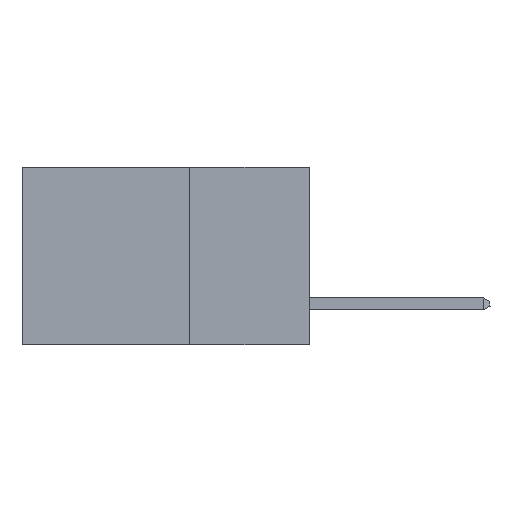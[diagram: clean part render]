
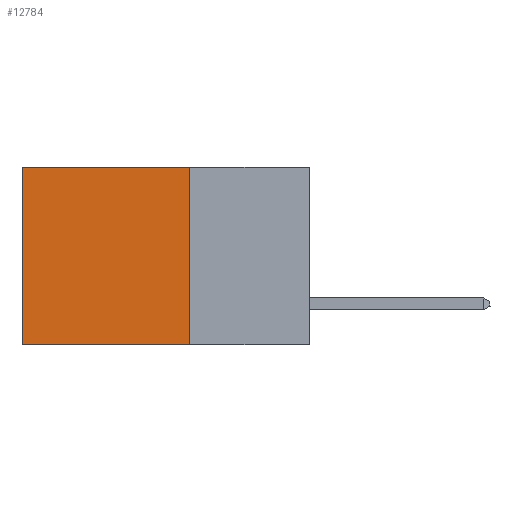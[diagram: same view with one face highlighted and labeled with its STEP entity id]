
A CAD part, left-side view. The second image highlights one B-rep face of the part: STEP entity #12784.
In plain terms, the highlighted planar face has unit normal (-1, 0, 0).
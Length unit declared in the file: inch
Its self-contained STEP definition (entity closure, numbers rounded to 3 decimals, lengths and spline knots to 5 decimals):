
#318 = EDGE_CURVE ( 'NONE', #12839, #1409, #3065, .T. ) ;
#541 = VECTOR ( 'NONE', #3881, 39.37008 ) ;
#1409 = VERTEX_POINT ( 'NONE', #2378 ) ;
#1896 = DIRECTION ( 'NONE',  ( 0., 1., 0. ) ) ;
#2196 = CARTESIAN_POINT ( 'NONE',  ( 0.2875, 0.25, 0. ) ) ;
#2378 = CARTESIAN_POINT ( 'NONE',  ( 0.2875, 0.6, -0.37 ) ) ;
#2907 = LINE ( 'NONE', #13317, #11770 ) ;
#3065 = LINE ( 'NONE', #16503, #20338 ) ;
#3502 = EDGE_LOOP ( 'NONE', ( #15024, #5044, #19921, #14026 ) ) ;
#3881 = DIRECTION ( 'NONE',  ( 0., 0., -1. ) ) ;
#5044 = ORIENTED_EDGE ( 'NONE', *, *, #7681, .F. ) ;
#6520 = DIRECTION ( 'NONE',  ( 0., 0., -1. ) ) ;
#7225 = AXIS2_PLACEMENT_3D ( 'NONE', #13760, #9853, #7696 ) ;
#7401 = LINE ( 'NONE', #12942, #8440 ) ;
#7681 = EDGE_CURVE ( 'NONE', #14162, #1409, #7401, .T. ) ;
#7696 = DIRECTION ( 'NONE',  ( 0., 0., -1. ) ) ;
#8440 = VECTOR ( 'NONE', #1896, 39.37008 ) ;
#9853 = DIRECTION ( 'NONE',  ( 1., 0., 0. ) ) ;
#11494 = DIRECTION ( 'NONE',  ( 0., 1., 0. ) ) ;
#11770 = VECTOR ( 'NONE', #11494, 39.37008 ) ;
#12561 = VERTEX_POINT ( 'NONE', #13825 ) ;
#12784 = ADVANCED_FACE ( 'NONE', ( #17078 ), #19588, .F. ) ;
#12839 = VERTEX_POINT ( 'NONE', #15323 ) ;
#12942 = CARTESIAN_POINT ( 'NONE',  ( 0.2875, 0.25, -0.37 ) ) ;
#13317 = CARTESIAN_POINT ( 'NONE',  ( 0.2875, 0.25, 0. ) ) ;
#13660 = EDGE_CURVE ( 'NONE', #12561, #14162, #18843, .T. ) ;
#13760 = CARTESIAN_POINT ( 'NONE',  ( 0.2875, 0.25, 0. ) ) ;
#13825 = CARTESIAN_POINT ( 'NONE',  ( 0.2875, 0.25, 0. ) ) ;
#14026 = ORIENTED_EDGE ( 'NONE', *, *, #18301, .T. ) ;
#14086 = CARTESIAN_POINT ( 'NONE',  ( 0.2875, 0.25, -0.37 ) ) ;
#14162 = VERTEX_POINT ( 'NONE', #14086 ) ;
#15024 = ORIENTED_EDGE ( 'NONE', *, *, #318, .T. ) ;
#15323 = CARTESIAN_POINT ( 'NONE',  ( 0.2875, 0.6, 0. ) ) ;
#16503 = CARTESIAN_POINT ( 'NONE',  ( 0.2875, 0.6, 0. ) ) ;
#17078 = FACE_OUTER_BOUND ( 'NONE', #3502, .T. ) ;
#18301 = EDGE_CURVE ( 'NONE', #12561, #12839, #2907, .T. ) ;
#18843 = LINE ( 'NONE', #2196, #541 ) ;
#19588 = PLANE ( 'NONE',  #7225 ) ;
#19921 = ORIENTED_EDGE ( 'NONE', *, *, #13660, .F. ) ;
#20338 = VECTOR ( 'NONE', #6520, 39.37008 ) ;
